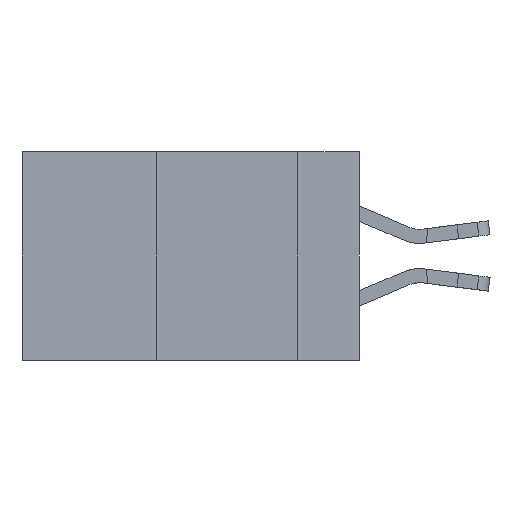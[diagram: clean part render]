
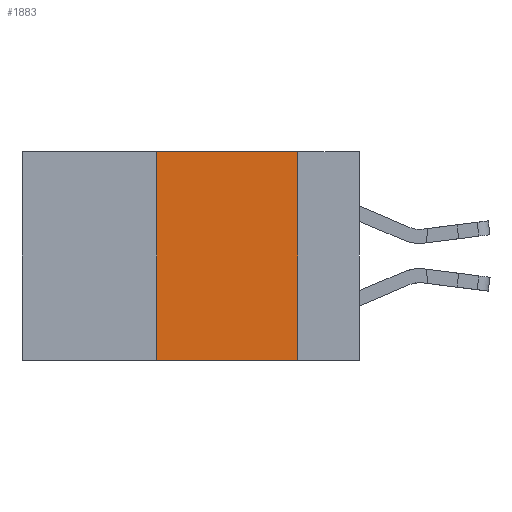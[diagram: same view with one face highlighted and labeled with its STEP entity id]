
A CAD part, left-side view. The second image highlights one B-rep face of the part: STEP entity #1883.
In plain terms, the highlighted planar face has unit normal (-1, 0, 0).
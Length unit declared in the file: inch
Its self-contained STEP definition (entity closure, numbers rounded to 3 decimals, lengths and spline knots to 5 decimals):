
#167 = ORIENTED_EDGE ( 'NONE', *, *, #3609, .F. ) ;
#932 = VERTEX_POINT ( 'NONE', #15004 ) ;
#1883 = ADVANCED_FACE ( 'NONE', ( #6608 ), #12278, .F. ) ;
#1936 = VECTOR ( 'NONE', #19063, 39.37008 ) ;
#2422 = DIRECTION ( 'NONE',  ( 0., -1., 0. ) ) ;
#2843 = EDGE_LOOP ( 'NONE', ( #6293, #9031, #167, #21500 ) ) ;
#3609 = EDGE_CURVE ( 'NONE', #932, #19954, #7955, .T. ) ;
#4694 = DIRECTION ( 'NONE',  ( 0., 0., -1. ) ) ;
#4859 = AXIS2_PLACEMENT_3D ( 'NONE', #17548, #19406, #4694 ) ;
#5568 = CARTESIAN_POINT ( 'NONE',  ( 0., 0.6, -0.37 ) ) ;
#5597 = CARTESIAN_POINT ( 'NONE',  ( 0., 0.11, -0.37 ) ) ;
#6011 = EDGE_CURVE ( 'NONE', #932, #13695, #20107, .T. ) ;
#6293 = ORIENTED_EDGE ( 'NONE', *, *, #9399, .F. ) ;
#6608 = FACE_OUTER_BOUND ( 'NONE', #2843, .T. ) ;
#7015 = CARTESIAN_POINT ( 'NONE',  ( 0., 0.36, 0. ) ) ;
#7064 = DIRECTION ( 'NONE',  ( 0., 0., 1. ) ) ;
#7955 = LINE ( 'NONE', #7015, #16560 ) ;
#9031 = ORIENTED_EDGE ( 'NONE', *, *, #14847, .F. ) ;
#9399 = EDGE_CURVE ( 'NONE', #15288, #13695, #10708, .T. ) ;
#10708 = LINE ( 'NONE', #10854, #14750 ) ;
#10854 = CARTESIAN_POINT ( 'NONE',  ( 0., 0.11, 0. ) ) ;
#10936 = DIRECTION ( 'NONE',  ( 0., 0., -1. ) ) ;
#12278 = PLANE ( 'NONE',  #4859 ) ;
#13657 = CARTESIAN_POINT ( 'NONE',  ( 0., 0.11, 0. ) ) ;
#13695 = VERTEX_POINT ( 'NONE', #5597 ) ;
#14750 = VECTOR ( 'NONE', #10936, 39.37008 ) ;
#14847 = EDGE_CURVE ( 'NONE', #19954, #15288, #15918, .T. ) ;
#15004 = CARTESIAN_POINT ( 'NONE',  ( 0., 0.36, -0.37 ) ) ;
#15288 = VERTEX_POINT ( 'NONE', #13657 ) ;
#15685 = VECTOR ( 'NONE', #2422, 39.37008 ) ;
#15918 = LINE ( 'NONE', #20623, #1936 ) ;
#16560 = VECTOR ( 'NONE', #7064, 39.37008 ) ;
#17548 = CARTESIAN_POINT ( 'NONE',  ( 0., 0.6, 0. ) ) ;
#19063 = DIRECTION ( 'NONE',  ( 0., -1., 0. ) ) ;
#19406 = DIRECTION ( 'NONE',  ( 1., 0., 0. ) ) ;
#19954 = VERTEX_POINT ( 'NONE', #21946 ) ;
#20107 = LINE ( 'NONE', #5568, #15685 ) ;
#20623 = CARTESIAN_POINT ( 'NONE',  ( 0., 0.6, 0. ) ) ;
#21500 = ORIENTED_EDGE ( 'NONE', *, *, #6011, .T. ) ;
#21946 = CARTESIAN_POINT ( 'NONE',  ( 0., 0.36, 0. ) ) ;
